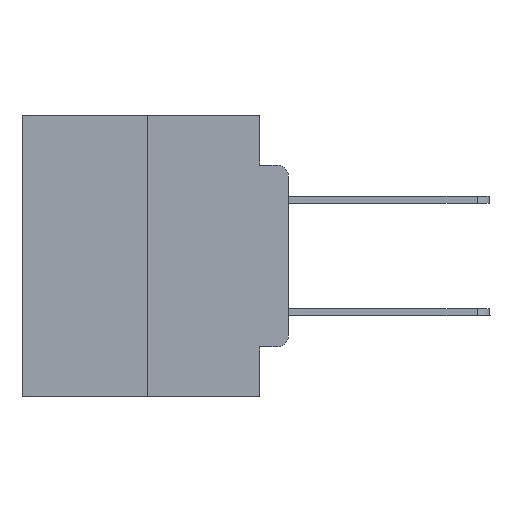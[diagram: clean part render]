
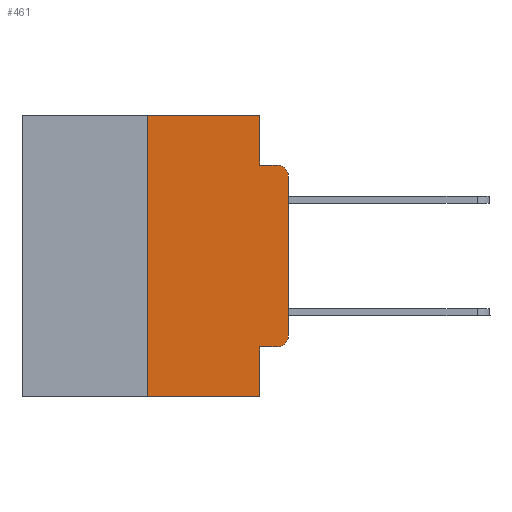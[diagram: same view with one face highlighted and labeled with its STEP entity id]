
A CAD part, left-side view. The second image highlights one B-rep face of the part: STEP entity #461.
In plain terms, the highlighted planar face has unit normal (-1, 0, 0).
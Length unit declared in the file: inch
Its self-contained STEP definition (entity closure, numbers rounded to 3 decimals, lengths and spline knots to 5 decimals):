
#272 = CARTESIAN_POINT ( 'NONE',  ( 0., 0.051, 0. ) ) ;
#273 = EDGE_CURVE ( 'NONE', #12031, #13581, #22486, .T. ) ;
#461 = ADVANCED_FACE ( 'NONE', ( #11302 ), #17503, .F. ) ;
#549 = VERTEX_POINT ( 'NONE', #2726 ) ;
#702 = DIRECTION ( 'NONE',  ( 0., -1., 0. ) ) ;
#745 = DIRECTION ( 'NONE',  ( 0., 0., -1. ) ) ;
#794 = CARTESIAN_POINT ( 'NONE',  ( 0., 0.02, -0.4115 ) ) ;
#1142 = ORIENTED_EDGE ( 'NONE', *, *, #3845, .F. ) ;
#1216 = CARTESIAN_POINT ( 'NONE',  ( 0., 0.051, 0. ) ) ;
#1644 = CIRCLE ( 'NONE', #5226, 0.02 ) ;
#1955 = DIRECTION ( 'NONE',  ( 0., 0., -1. ) ) ;
#2274 = EDGE_CURVE ( 'NONE', #7876, #549, #1644, .T. ) ;
#2445 = CARTESIAN_POINT ( 'NONE',  ( 0., 0.473, 0. ) ) ;
#2726 = CARTESIAN_POINT ( 'NONE',  ( 0., 0., -0.3915 ) ) ;
#2988 = CARTESIAN_POINT ( 'NONE',  ( 0., 0., 0. ) ) ;
#2995 = VERTEX_POINT ( 'NONE', #4883 ) ;
#3119 = LINE ( 'NONE', #2988, #3982 ) ;
#3555 = DIRECTION ( 'NONE',  ( 0., 0., -1. ) ) ;
#3845 = EDGE_CURVE ( 'NONE', #2995, #18789, #23689, .T. ) ;
#3982 = VECTOR ( 'NONE', #11571, 39.37008 ) ;
#4092 = LINE ( 'NONE', #12680, #8120 ) ;
#4655 = DIRECTION ( 'NONE',  ( 0., -1., 0. ) ) ;
#4730 = LINE ( 'NONE', #15010, #5437 ) ;
#4883 = CARTESIAN_POINT ( 'NONE',  ( 0., 0.25, 0. ) ) ;
#4960 = ORIENTED_EDGE ( 'NONE', *, *, #13309, .F. ) ;
#4967 = DIRECTION ( 'NONE',  ( 1., 0., 0. ) ) ;
#5226 = AXIS2_PLACEMENT_3D ( 'NONE', #23135, #9906, #3555 ) ;
#5437 = VECTOR ( 'NONE', #6972, 39.37008 ) ;
#5923 = EDGE_LOOP ( 'NONE', ( #15816, #17467, #11656, #6422, #1142, #4960, #22776, #19930, #15067, #22312 ) ) ;
#5928 = CARTESIAN_POINT ( 'NONE',  ( 0., 0.25, -0.5 ) ) ;
#6239 = DIRECTION ( 'NONE',  ( 0., 0., -1. ) ) ;
#6422 = ORIENTED_EDGE ( 'NONE', *, *, #17214, .F. ) ;
#6972 = DIRECTION ( 'NONE',  ( 0., 0., 1. ) ) ;
#7876 = VERTEX_POINT ( 'NONE', #794 ) ;
#8120 = VECTOR ( 'NONE', #4655, 39.37008 ) ;
#8655 = VECTOR ( 'NONE', #22163, 39.37008 ) ;
#8776 = DIRECTION ( 'NONE',  ( 0., -1., 0. ) ) ;
#9411 = LINE ( 'NONE', #22238, #9913 ) ;
#9906 = DIRECTION ( 'NONE',  ( -1., 0., 0. ) ) ;
#9913 = VECTOR ( 'NONE', #702, 39.37008 ) ;
#11302 = FACE_OUTER_BOUND ( 'NONE', #5923, .T. ) ;
#11571 = DIRECTION ( 'NONE',  ( 0., 0., 1. ) ) ;
#11656 = ORIENTED_EDGE ( 'NONE', *, *, #25574, .F. ) ;
#12031 = VERTEX_POINT ( 'NONE', #27418 ) ;
#12589 = AXIS2_PLACEMENT_3D ( 'NONE', #14976, #23283, #6239 ) ;
#12680 = CARTESIAN_POINT ( 'NONE',  ( 0., 0.473, -0.5 ) ) ;
#12748 = EDGE_CURVE ( 'NONE', #21050, #20619, #4092, .T. ) ;
#12896 = EDGE_CURVE ( 'NONE', #22525, #7876, #9411, .T. ) ;
#12978 = CARTESIAN_POINT ( 'NONE',  ( 0., 0.473, 0. ) ) ;
#13309 = EDGE_CURVE ( 'NONE', #21050, #2995, #4730, .T. ) ;
#13581 = VERTEX_POINT ( 'NONE', #18494 ) ;
#14976 = CARTESIAN_POINT ( 'NONE',  ( 0., 0.02, -0.1085 ) ) ;
#15010 = CARTESIAN_POINT ( 'NONE',  ( 0., 0.25, 0. ) ) ;
#15067 = ORIENTED_EDGE ( 'NONE', *, *, #12896, .T. ) ;
#15816 = ORIENTED_EDGE ( 'NONE', *, *, #24247, .T. ) ;
#16338 = EDGE_CURVE ( 'NONE', #22525, #20619, #25308, .T. ) ;
#17214 = EDGE_CURVE ( 'NONE', #18789, #23559, #21238, .T. ) ;
#17467 = ORIENTED_EDGE ( 'NONE', *, *, #273, .T. ) ;
#17503 = PLANE ( 'NONE',  #22065 ) ;
#18349 = CARTESIAN_POINT ( 'NONE',  ( 0., 0.051, -0.5 ) ) ;
#18494 = CARTESIAN_POINT ( 'NONE',  ( 0., 0.02, -0.0885 ) ) ;
#18789 = VERTEX_POINT ( 'NONE', #1216 ) ;
#18951 = CARTESIAN_POINT ( 'NONE',  ( 0., 0.051, 0. ) ) ;
#19489 = LINE ( 'NONE', #19757, #26074 ) ;
#19757 = CARTESIAN_POINT ( 'NONE',  ( 0., 0.051, -0.0885 ) ) ;
#19882 = DIRECTION ( 'NONE',  ( 0., -1., 0. ) ) ;
#19930 = ORIENTED_EDGE ( 'NONE', *, *, #16338, .F. ) ;
#20619 = VERTEX_POINT ( 'NONE', #18349 ) ;
#21050 = VERTEX_POINT ( 'NONE', #5928 ) ;
#21238 = LINE ( 'NONE', #272, #22191 ) ;
#22065 = AXIS2_PLACEMENT_3D ( 'NONE', #2445, #4967, #745 ) ;
#22163 = DIRECTION ( 'NONE',  ( 0., 0., -1. ) ) ;
#22191 = VECTOR ( 'NONE', #1955, 39.37008 ) ;
#22238 = CARTESIAN_POINT ( 'NONE',  ( 0., 0.051, -0.4115 ) ) ;
#22312 = ORIENTED_EDGE ( 'NONE', *, *, #2274, .T. ) ;
#22486 = CIRCLE ( 'NONE', #12589, 0.02 ) ;
#22525 = VERTEX_POINT ( 'NONE', #22586 ) ;
#22586 = CARTESIAN_POINT ( 'NONE',  ( 0., 0.051, -0.4115 ) ) ;
#22776 = ORIENTED_EDGE ( 'NONE', *, *, #12748, .T. ) ;
#23135 = CARTESIAN_POINT ( 'NONE',  ( 0., 0.02, -0.3915 ) ) ;
#23283 = DIRECTION ( 'NONE',  ( -1., 0., 0. ) ) ;
#23559 = VERTEX_POINT ( 'NONE', #27672 ) ;
#23689 = LINE ( 'NONE', #12978, #25880 ) ;
#24247 = EDGE_CURVE ( 'NONE', #549, #12031, #3119, .T. ) ;
#25308 = LINE ( 'NONE', #18951, #8655 ) ;
#25574 = EDGE_CURVE ( 'NONE', #23559, #13581, #19489, .T. ) ;
#25880 = VECTOR ( 'NONE', #19882, 39.37008 ) ;
#26074 = VECTOR ( 'NONE', #8776, 39.37008 ) ;
#27418 = CARTESIAN_POINT ( 'NONE',  ( 0., 0., -0.1085 ) ) ;
#27672 = CARTESIAN_POINT ( 'NONE',  ( 0., 0.051, -0.0885 ) ) ;
